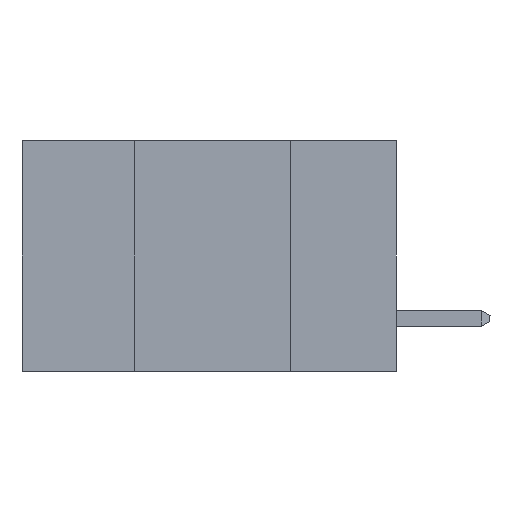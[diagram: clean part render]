
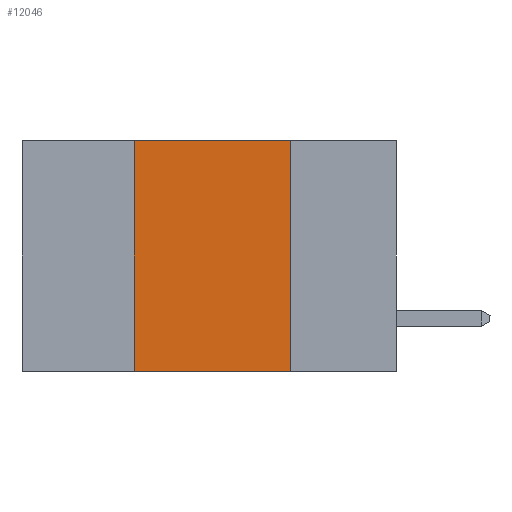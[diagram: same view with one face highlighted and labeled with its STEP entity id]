
A CAD part, left-side view. The second image highlights one B-rep face of the part: STEP entity #12046.
In plain terms, the highlighted planar face has unit normal (-1, 0, 0).
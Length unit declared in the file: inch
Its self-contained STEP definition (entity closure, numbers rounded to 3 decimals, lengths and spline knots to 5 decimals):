
#507 = PLANE ( 'NONE',  #19629 ) ;
#1350 = EDGE_CURVE ( 'NONE', #2254, #7280, #16229, .T. ) ;
#1695 = CARTESIAN_POINT ( 'NONE',  ( 0., 0.17, -0.37 ) ) ;
#1904 = LINE ( 'NONE', #10109, #14638 ) ;
#1933 = ORIENTED_EDGE ( 'NONE', *, *, #1350, .F. ) ;
#2020 = DIRECTION ( 'NONE',  ( 0., -1., 0. ) ) ;
#2254 = VERTEX_POINT ( 'NONE', #16178 ) ;
#2374 = CARTESIAN_POINT ( 'NONE',  ( 0., 0.17, 0. ) ) ;
#2627 = VECTOR ( 'NONE', #17290, 39.37008 ) ;
#3359 = EDGE_CURVE ( 'NONE', #14218, #4284, #9480, .T. ) ;
#3593 = CARTESIAN_POINT ( 'NONE',  ( 0., 0.6, 0. ) ) ;
#3967 = EDGE_LOOP ( 'NONE', ( #6712, #4149, #1933, #11457 ) ) ;
#4149 = ORIENTED_EDGE ( 'NONE', *, *, #9977, .F. ) ;
#4284 = VERTEX_POINT ( 'NONE', #19171 ) ;
#5909 = CARTESIAN_POINT ( 'NONE',  ( 0., 0.6, -0.37 ) ) ;
#6712 = ORIENTED_EDGE ( 'NONE', *, *, #3359, .F. ) ;
#7280 = VERTEX_POINT ( 'NONE', #14561 ) ;
#9480 = LINE ( 'NONE', #1695, #16971 ) ;
#9977 = EDGE_CURVE ( 'NONE', #7280, #14218, #1904, .T. ) ;
#10089 = DIRECTION ( 'NONE',  ( 1., 0., 0. ) ) ;
#10109 = CARTESIAN_POINT ( 'NONE',  ( 0., 0.6, 0. ) ) ;
#10260 = VECTOR ( 'NONE', #21024, 39.37008 ) ;
#11457 = ORIENTED_EDGE ( 'NONE', *, *, #15081, .T. ) ;
#12046 = ADVANCED_FACE ( 'NONE', ( #18179 ), #507, .F. ) ;
#12768 = DIRECTION ( 'NONE',  ( 0., 0., -1. ) ) ;
#13478 = DIRECTION ( 'NONE',  ( 0., 0., -1. ) ) ;
#14218 = VERTEX_POINT ( 'NONE', #2374 ) ;
#14561 = CARTESIAN_POINT ( 'NONE',  ( 0., 0.42, 0. ) ) ;
#14638 = VECTOR ( 'NONE', #2020, 39.37008 ) ;
#15081 = EDGE_CURVE ( 'NONE', #2254, #4284, #16983, .T. ) ;
#16178 = CARTESIAN_POINT ( 'NONE',  ( 0., 0.42, -0.37 ) ) ;
#16229 = LINE ( 'NONE', #17510, #10260 ) ;
#16971 = VECTOR ( 'NONE', #12768, 39.37008 ) ;
#16983 = LINE ( 'NONE', #5909, #2627 ) ;
#17290 = DIRECTION ( 'NONE',  ( 0., -1., 0. ) ) ;
#17510 = CARTESIAN_POINT ( 'NONE',  ( 0., 0.42, -0.37 ) ) ;
#18179 = FACE_OUTER_BOUND ( 'NONE', #3967, .T. ) ;
#19171 = CARTESIAN_POINT ( 'NONE',  ( 0., 0.17, -0.37 ) ) ;
#19629 = AXIS2_PLACEMENT_3D ( 'NONE', #3593, #10089, #13478 ) ;
#21024 = DIRECTION ( 'NONE',  ( 0., 0., 1. ) ) ;
